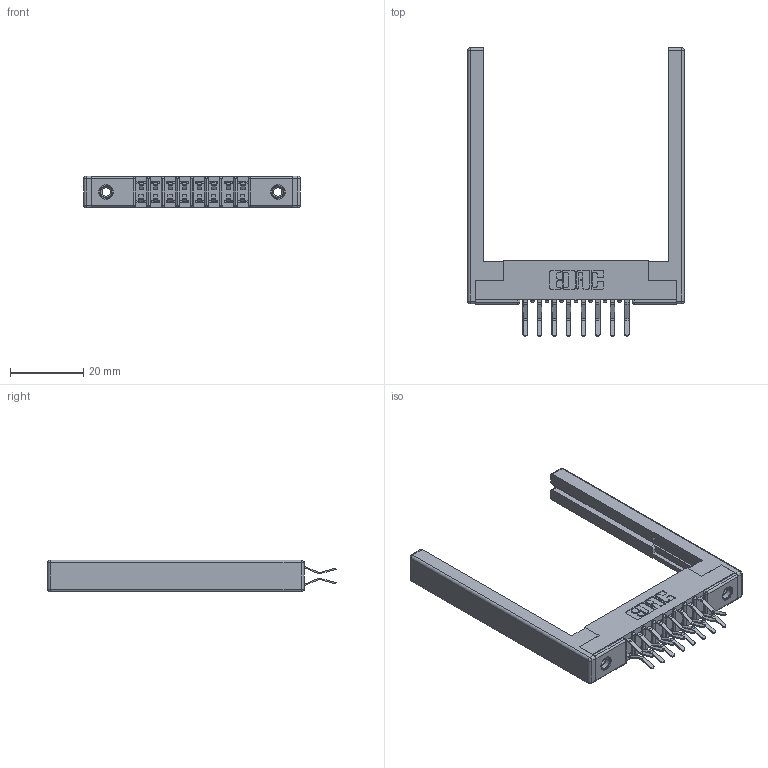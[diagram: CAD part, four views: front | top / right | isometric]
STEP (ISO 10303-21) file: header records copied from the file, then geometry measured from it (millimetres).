
FILE_DESCRIPTION (( 'STEP AP203' ), '1' );
FILE_NAME ('357-016-460-268.STEP', '2020-10-02T19:55:42', ( '' ), ( '' ), 'SwSTEP 2.0', 'SolidWorks 2020', '' );
FILE_SCHEMA (( 'CONFIG_CONTROL_DESIGN' ));
Length unit declared in the file: inch
Products named in the file (5): 307-290-001_560; 307 Part_.156 Dia Mounting Holes; 307-220-068; 345-250-001_345-250-001-102; 357-016-460-268
Assembly tree (21 placements, depth 2):
  357-016-460-268
    307 Part_.156 Dia Mounting Holes
    307-290-001_560  x16
    307-220-068  x2
    345-250-001_345-250-001-102  x2
Bounding box: 59.13 x 78.69 x 8.71 mm (x, y, z)
Volume: 8450.8 mm3; surface area: 10304.4 mm2
Topology: 21 solids, 21 shells, 1081 faces, 2985 edges, 1922 vertices
Faces by surface type: plane 686, cylinder 353, sphere 26, cone 12, torus 4
Entity records: 14169 total; most frequent: CARTESIAN_POINT 2305, DIRECTION 2288, ORIENTED_EDGE 2272, EDGE_CURVE 1136, VECTOR 854, LINE 854, VERTEX_POINT 734, AXIS2_PLACEMENT_3D 717
